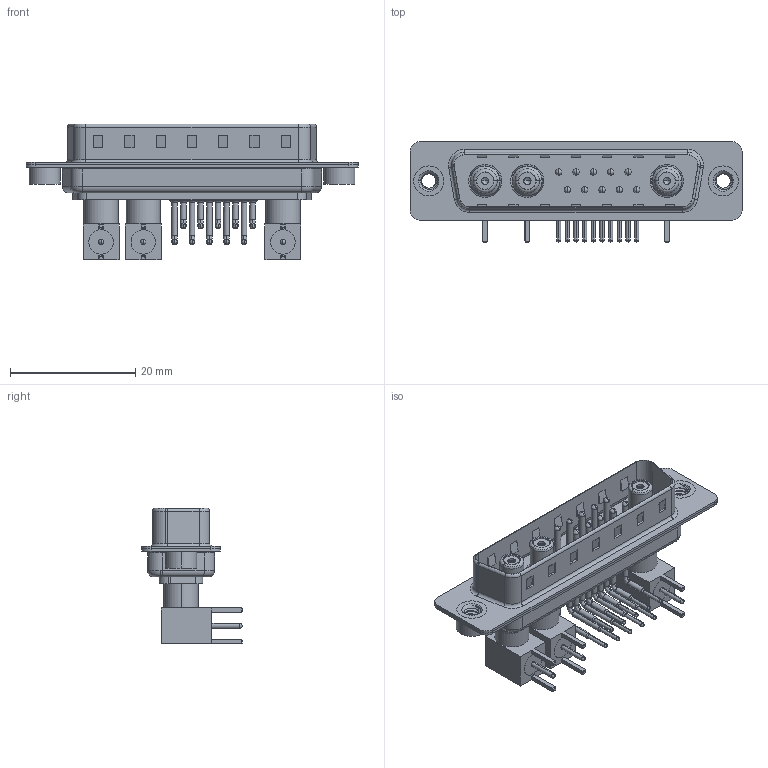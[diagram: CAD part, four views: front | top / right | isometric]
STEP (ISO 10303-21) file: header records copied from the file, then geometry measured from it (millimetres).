
FILE_DESCRIPTION (( 'STEP AP203' ), '1' );
FILE_NAME ('629-13W3240-5T2.STEP', '2022-05-10T02:22:56', ( '' ), ( '' ), 'SwSTEP 2.0', 'SolidWorks 2020', '' );
FILE_SCHEMA (( 'CONFIG_CONTROL_DESIGN' ));
Length unit declared in the file: millimetre
Products named in the file (17): Insulator Socket 2; 629Combo Shell Front_25 Contacts; Insulator Socket; 629-13W3240-5T2; Socket_RA; 629Combo Contact Row 2; RA Back Shell; 629Combo Threaded Rivet_2; 629Combo Shell Rear_25 Contacts; Co-Ax Jack Assy_RA; Locking Collar; Insulator RA Pin; 629Combo Housing_13W3; 629Combo Contact Row 1; Co-Ax Jack_RA PC Tail
Assembly tree (39 placements, depth 3):
  629-13W3240-5T2
    629Combo Housing_13W3
    629Combo Shell Rear_25 Contacts
    629Combo Shell Front_25 Contacts
    629Combo Threaded Rivet_2  x2
    Co-Ax Jack Assy_RA
      Co-Ax Jack_RA PC Tail
      Insulator Socket
      Insulator Socket 2
      Locking Collar
      Socket_RA
      RA Back Shell
      Insulator RA Pin
    Co-Ax Jack Assy_RA
      Co-Ax Jack_RA PC Tail
      Insulator Socket
      Insulator Socket 2
      Locking Collar
      Socket_RA
      RA Back Shell
      Insulator RA Pin
    Co-Ax Jack Assy_RA
      Co-Ax Jack_RA PC Tail
      Insulator Socket
      Insulator Socket 2
      Locking Collar
      Socket_RA
      RA Back Shell
      Insulator RA Pin
    629Combo Contact Row 1  x5
    629Combo Contact Row 2  x5
Bounding box: 53.05 x 16 x 21.71 mm (x, y, z)
Volume: 3655.8 mm3; surface area: 9904.6 mm2
Topology: 36 solids, 36 shells, 1932 faces, 5102 edges, 3271 vertices
Faces by surface type: plane 982, cylinder 698, cone 109, bspline 69, torus 68, sphere 6
Entity records: 28132 total; most frequent: CARTESIAN_POINT 6014, DIRECTION 4298, ORIENTED_EDGE 3982, EDGE_CURVE 1991, AXIS2_PLACEMENT_3D 1554, VERTEX_POINT 1279, LINE 1190, VECTOR 1190
